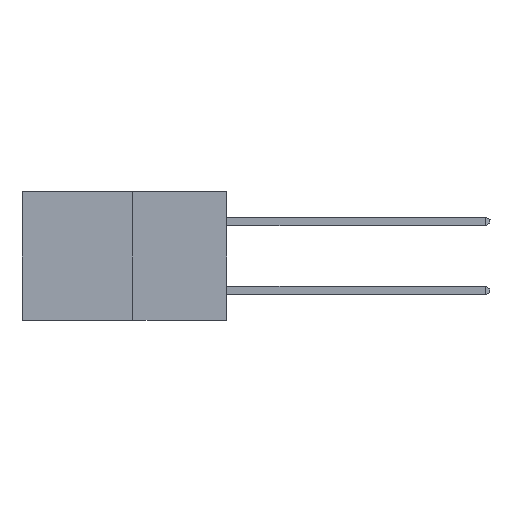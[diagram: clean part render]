
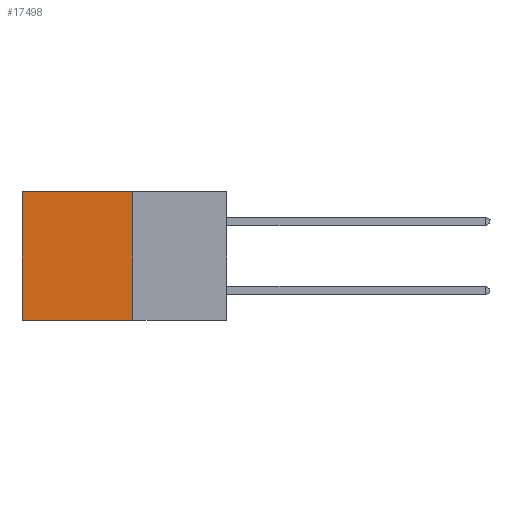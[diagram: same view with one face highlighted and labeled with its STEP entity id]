
A CAD part, left-side view. The second image highlights one B-rep face of the part: STEP entity #17498.
In plain terms, the highlighted planar face has unit normal (-1, 0, 0).
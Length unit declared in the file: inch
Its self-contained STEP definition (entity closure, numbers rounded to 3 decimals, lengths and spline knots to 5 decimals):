
#904 = PLANE ( 'NONE',  #16930 ) ;
#1558 = LINE ( 'NONE', #3542, #11289 ) ;
#2907 = DIRECTION ( 'NONE',  ( 0., 0., -1. ) ) ;
#3542 = CARTESIAN_POINT ( 'NONE',  ( 0.277, 0.27, 0. ) ) ;
#3760 = LINE ( 'NONE', #20674, #18455 ) ;
#4246 = FACE_OUTER_BOUND ( 'NONE', #16342, .T. ) ;
#4253 = VECTOR ( 'NONE', #14289, 39.37008 ) ;
#4855 = LINE ( 'NONE', #14428, #4253 ) ;
#4915 = CARTESIAN_POINT ( 'NONE',  ( 0.277, 0.59, -0.37 ) ) ;
#5053 = LINE ( 'NONE', #4915, #23538 ) ;
#5894 = EDGE_CURVE ( 'NONE', #14492, #14466, #4855, .T. ) ;
#6019 = ORIENTED_EDGE ( 'NONE', *, *, #14720, .T. ) ;
#9284 = ORIENTED_EDGE ( 'NONE', *, *, #10099, .T. ) ;
#9297 = EDGE_CURVE ( 'NONE', #24271, #14492, #3760, .T. ) ;
#10099 = EDGE_CURVE ( 'NONE', #24271, #21008, #1558, .T. ) ;
#11181 = DIRECTION ( 'NONE',  ( 0., 1., 0. ) ) ;
#11289 = VECTOR ( 'NONE', #11181, 39.37008 ) ;
#11480 = ORIENTED_EDGE ( 'NONE', *, *, #5894, .F. ) ;
#11490 = CARTESIAN_POINT ( 'NONE',  ( 0.277, 0.59, 0. ) ) ;
#12564 = CARTESIAN_POINT ( 'NONE',  ( 0.277, 0.27, -0.37 ) ) ;
#13045 = DIRECTION ( 'NONE',  ( 0., 0., -1. ) ) ;
#14289 = DIRECTION ( 'NONE',  ( 0., 1., 0. ) ) ;
#14428 = CARTESIAN_POINT ( 'NONE',  ( 0.277, 0.27, -0.37 ) ) ;
#14465 = DIRECTION ( 'NONE',  ( 1., 0., 0. ) ) ;
#14466 = VERTEX_POINT ( 'NONE', #21379 ) ;
#14492 = VERTEX_POINT ( 'NONE', #23363 ) ;
#14720 = EDGE_CURVE ( 'NONE', #21008, #14466, #5053, .T. ) ;
#16342 = EDGE_LOOP ( 'NONE', ( #6019, #11480, #19380, #9284 ) ) ;
#16386 = DIRECTION ( 'NONE',  ( 0., 0., -1. ) ) ;
#16930 = AXIS2_PLACEMENT_3D ( 'NONE', #12564, #14465, #2907 ) ;
#17498 = ADVANCED_FACE ( 'NONE', ( #4246 ), #904, .F. ) ;
#18455 = VECTOR ( 'NONE', #13045, 39.37008 ) ;
#19380 = ORIENTED_EDGE ( 'NONE', *, *, #9297, .F. ) ;
#20674 = CARTESIAN_POINT ( 'NONE',  ( 0.277, 0.27, -0.37 ) ) ;
#21008 = VERTEX_POINT ( 'NONE', #11490 ) ;
#21379 = CARTESIAN_POINT ( 'NONE',  ( 0.277, 0.59, -0.37 ) ) ;
#22798 = CARTESIAN_POINT ( 'NONE',  ( 0.277, 0.27, 0. ) ) ;
#23363 = CARTESIAN_POINT ( 'NONE',  ( 0.277, 0.27, -0.37 ) ) ;
#23538 = VECTOR ( 'NONE', #16386, 39.37008 ) ;
#24271 = VERTEX_POINT ( 'NONE', #22798 ) ;
